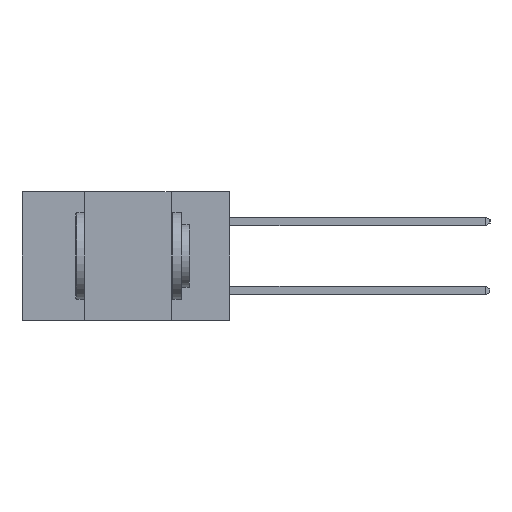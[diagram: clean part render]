
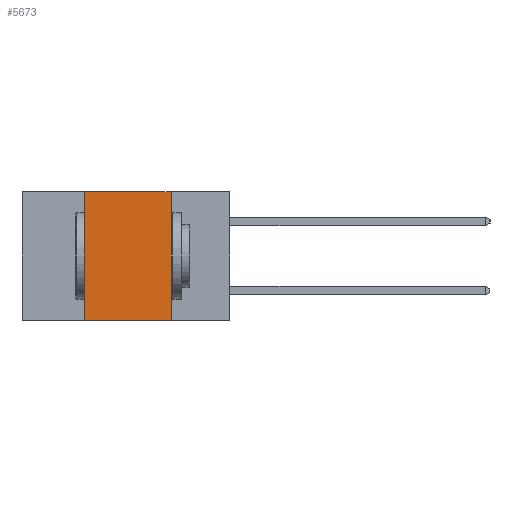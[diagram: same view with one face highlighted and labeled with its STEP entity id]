
A CAD part, left-side view. The second image highlights one B-rep face of the part: STEP entity #5673.
In plain terms, the highlighted planar face has unit normal (-1, 0, 0).
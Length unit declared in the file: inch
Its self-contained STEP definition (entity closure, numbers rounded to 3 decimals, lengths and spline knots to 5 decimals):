
#283 = DIRECTION ( 'NONE',  ( 0., -1., 0. ) ) ;
#771 = CARTESIAN_POINT ( 'NONE',  ( 0., 0.42, 0. ) ) ;
#1234 = EDGE_CURVE ( 'NONE', #8063, #15197, #18184, .T. ) ;
#1635 = LINE ( 'NONE', #5225, #9432 ) ;
#1991 = LINE ( 'NONE', #11488, #6166 ) ;
#2600 = VECTOR ( 'NONE', #10092, 39.37008 ) ;
#2686 = ORIENTED_EDGE ( 'NONE', *, *, #19433, .T. ) ;
#4218 = DIRECTION ( 'NONE',  ( 0., 0., -1. ) ) ;
#4321 = DIRECTION ( 'NONE',  ( 1., 0., 0. ) ) ;
#4328 = CARTESIAN_POINT ( 'NONE',  ( 0., 0.6, 0. ) ) ;
#4518 = VERTEX_POINT ( 'NONE', #12879 ) ;
#4632 = AXIS2_PLACEMENT_3D ( 'NONE', #4328, #4321, #4218 ) ;
#5225 = CARTESIAN_POINT ( 'NONE',  ( 0., 0.6, -0.37 ) ) ;
#5673 = ADVANCED_FACE ( 'NONE', ( #11395 ), #5850, .F. ) ;
#5850 = PLANE ( 'NONE',  #4632 ) ;
#6166 = VECTOR ( 'NONE', #283, 39.37008 ) ;
#6762 = DIRECTION ( 'NONE',  ( 0., -1., 0. ) ) ;
#7886 = ORIENTED_EDGE ( 'NONE', *, *, #8001, .F. ) ;
#8001 = EDGE_CURVE ( 'NONE', #8226, #8063, #1991, .T. ) ;
#8063 = VERTEX_POINT ( 'NONE', #11164 ) ;
#8226 = VERTEX_POINT ( 'NONE', #771 ) ;
#9432 = VECTOR ( 'NONE', #6762, 39.37008 ) ;
#10092 = DIRECTION ( 'NONE',  ( 0., 0., -1. ) ) ;
#10106 = CARTESIAN_POINT ( 'NONE',  ( 0., 0.17, 0. ) ) ;
#10325 = LINE ( 'NONE', #16030, #17718 ) ;
#10503 = ORIENTED_EDGE ( 'NONE', *, *, #1234, .F. ) ;
#11164 = CARTESIAN_POINT ( 'NONE',  ( 0., 0.17, 0. ) ) ;
#11395 = FACE_OUTER_BOUND ( 'NONE', #12450, .T. ) ;
#11488 = CARTESIAN_POINT ( 'NONE',  ( 0., 0.6, 0. ) ) ;
#11925 = EDGE_CURVE ( 'NONE', #4518, #8226, #10325, .T. ) ;
#12142 = CARTESIAN_POINT ( 'NONE',  ( 0., 0.17, -0.37 ) ) ;
#12450 = EDGE_LOOP ( 'NONE', ( #10503, #7886, #14065, #2686 ) ) ;
#12879 = CARTESIAN_POINT ( 'NONE',  ( 0., 0.42, -0.37 ) ) ;
#13087 = DIRECTION ( 'NONE',  ( 0., 0., 1. ) ) ;
#14065 = ORIENTED_EDGE ( 'NONE', *, *, #11925, .F. ) ;
#15197 = VERTEX_POINT ( 'NONE', #12142 ) ;
#16030 = CARTESIAN_POINT ( 'NONE',  ( 0., 0.42, 0. ) ) ;
#17718 = VECTOR ( 'NONE', #13087, 39.37008 ) ;
#18184 = LINE ( 'NONE', #10106, #2600 ) ;
#19433 = EDGE_CURVE ( 'NONE', #4518, #15197, #1635, .T. ) ;
